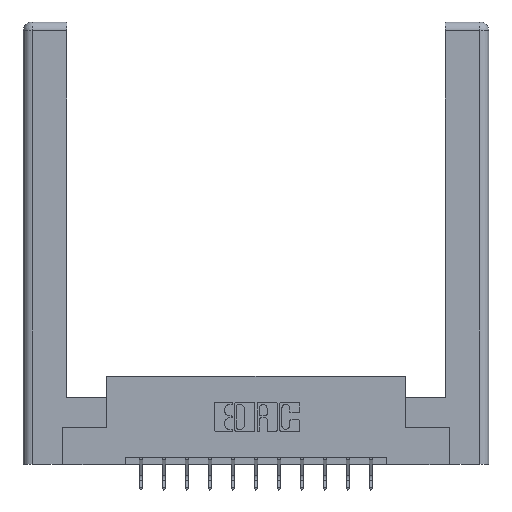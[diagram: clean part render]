
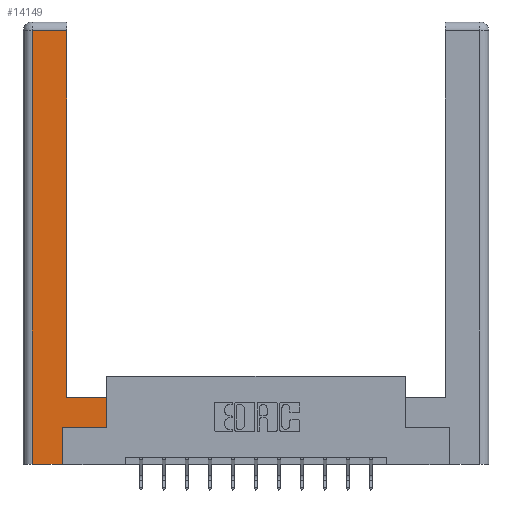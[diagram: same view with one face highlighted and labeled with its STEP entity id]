
A CAD part, top view. The second image highlights one B-rep face of the part: STEP entity #14149.
In plain terms, the highlighted planar face has unit normal (0, 0, 1).
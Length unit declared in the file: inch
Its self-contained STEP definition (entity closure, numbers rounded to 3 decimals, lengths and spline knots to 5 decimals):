
#106 = CARTESIAN_POINT ( 'NONE',  ( 0.295, 3., 0. ) ) ;
#637 = VECTOR ( 'NONE', #11066, 39.37008 ) ;
#917 = ORIENTED_EDGE ( 'NONE', *, *, #14812, .T. ) ;
#1295 = EDGE_CURVE ( 'NONE', #9927, #1397, #6082, .T. ) ;
#1319 = CARTESIAN_POINT ( 'NONE',  ( 0.295, 2.94, 0. ) ) ;
#1342 = EDGE_CURVE ( 'NONE', #3795, #6010, #13004, .T. ) ;
#1397 = VERTEX_POINT ( 'NONE', #7512 ) ;
#1559 = LINE ( 'NONE', #2731, #637 ) ;
#1615 = EDGE_CURVE ( 'NONE', #6010, #3502, #6625, .T. ) ;
#2273 = ORIENTED_EDGE ( 'NONE', *, *, #1615, .T. ) ;
#2372 = FACE_OUTER_BOUND ( 'NONE', #13453, .T. ) ;
#2423 = DIRECTION ( 'NONE',  ( 0., 1., 0. ) ) ;
#2568 = CARTESIAN_POINT ( 'NONE',  ( 0.565, 0.245, 0. ) ) ;
#2731 = CARTESIAN_POINT ( 'NONE',  ( 0.0615, 0., 0. ) ) ;
#2876 = VERTEX_POINT ( 'NONE', #3039 ) ;
#3039 = CARTESIAN_POINT ( 'NONE',  ( 0.0615, 0., 0. ) ) ;
#3061 = ORIENTED_EDGE ( 'NONE', *, *, #4952, .T. ) ;
#3245 = CARTESIAN_POINT ( 'NONE',  ( 0.0615, 2.94, 0. ) ) ;
#3275 = DIRECTION ( 'NONE',  ( -1., 0., 0. ) ) ;
#3372 = CARTESIAN_POINT ( 'NONE',  ( 0., 0., 0. ) ) ;
#3502 = VERTEX_POINT ( 'NONE', #7410 ) ;
#3795 = VERTEX_POINT ( 'NONE', #4969 ) ;
#3989 = LINE ( 'NONE', #4559, #9600 ) ;
#4398 = VECTOR ( 'NONE', #11523, 39.37008 ) ;
#4559 = CARTESIAN_POINT ( 'NONE',  ( 0.265, 0.245, 0. ) ) ;
#4767 = DIRECTION ( 'NONE',  ( 0., 1., 0. ) ) ;
#4783 = VECTOR ( 'NONE', #4767, 39.37008 ) ;
#4952 = EDGE_CURVE ( 'NONE', #1397, #2876, #1559, .T. ) ;
#4969 = CARTESIAN_POINT ( 'NONE',  ( 0.265, 0.245, 0. ) ) ;
#5210 = CARTESIAN_POINT ( 'NONE',  ( 0.265, 0., 0. ) ) ;
#5604 = PLANE ( 'NONE',  #13575 ) ;
#5936 = CARTESIAN_POINT ( 'NONE',  ( 0.295, 0.45, 0. ) ) ;
#6010 = VERTEX_POINT ( 'NONE', #2568 ) ;
#6082 = LINE ( 'NONE', #3245, #7016 ) ;
#6287 = EDGE_CURVE ( 'NONE', #2876, #15184, #9234, .T. ) ;
#6396 = ORIENTED_EDGE ( 'NONE', *, *, #6968, .T. ) ;
#6625 = LINE ( 'NONE', #9741, #4783 ) ;
#6968 = EDGE_CURVE ( 'NONE', #3502, #10598, #7924, .T. ) ;
#7016 = VECTOR ( 'NONE', #12784, 39.37008 ) ;
#7410 = CARTESIAN_POINT ( 'NONE',  ( 0.565, 0.45, 0. ) ) ;
#7420 = ORIENTED_EDGE ( 'NONE', *, *, #10641, .T. ) ;
#7512 = CARTESIAN_POINT ( 'NONE',  ( 0.0615, 2.94, 0. ) ) ;
#7924 = LINE ( 'NONE', #14308, #14082 ) ;
#8124 = DIRECTION ( 'NONE',  ( 0., 0., -1. ) ) ;
#8205 = VECTOR ( 'NONE', #2423, 39.37008 ) ;
#8293 = DIRECTION ( 'NONE',  ( 1., 0., 0. ) ) ;
#9234 = LINE ( 'NONE', #11367, #4398 ) ;
#9600 = VECTOR ( 'NONE', #15350, 39.37008 ) ;
#9741 = CARTESIAN_POINT ( 'NONE',  ( 0.565, 0.45, 0. ) ) ;
#9927 = VERTEX_POINT ( 'NONE', #1319 ) ;
#10598 = VERTEX_POINT ( 'NONE', #5936 ) ;
#10641 = EDGE_CURVE ( 'NONE', #10598, #9927, #11376, .T. ) ;
#11066 = DIRECTION ( 'NONE',  ( 0., -1., 0. ) ) ;
#11254 = ORIENTED_EDGE ( 'NONE', *, *, #6287, .T. ) ;
#11367 = CARTESIAN_POINT ( 'NONE',  ( 0.265, 0., 0. ) ) ;
#11376 = LINE ( 'NONE', #106, #8205 ) ;
#11523 = DIRECTION ( 'NONE',  ( 1., 0., 0. ) ) ;
#12784 = DIRECTION ( 'NONE',  ( -1., 0., 0. ) ) ;
#13004 = LINE ( 'NONE', #14258, #14321 ) ;
#13016 = ORIENTED_EDGE ( 'NONE', *, *, #1342, .T. ) ;
#13453 = EDGE_LOOP ( 'NONE', ( #7420, #14824, #3061, #11254, #917, #13016, #2273, #6396 ) ) ;
#13575 = AXIS2_PLACEMENT_3D ( 'NONE', #3372, #8124, #3275 ) ;
#14082 = VECTOR ( 'NONE', #14255, 39.37008 ) ;
#14149 = ADVANCED_FACE ( 'NONE', ( #2372 ), #5604, .F. ) ;
#14255 = DIRECTION ( 'NONE',  ( -1., 0., 0. ) ) ;
#14258 = CARTESIAN_POINT ( 'NONE',  ( 0.565, 0.245, 0. ) ) ;
#14308 = CARTESIAN_POINT ( 'NONE',  ( 0.295, 0.45, 0. ) ) ;
#14321 = VECTOR ( 'NONE', #8293, 39.37008 ) ;
#14812 = EDGE_CURVE ( 'NONE', #15184, #3795, #3989, .T. ) ;
#14824 = ORIENTED_EDGE ( 'NONE', *, *, #1295, .T. ) ;
#15184 = VERTEX_POINT ( 'NONE', #5210 ) ;
#15350 = DIRECTION ( 'NONE',  ( 0., 1., 0. ) ) ;
